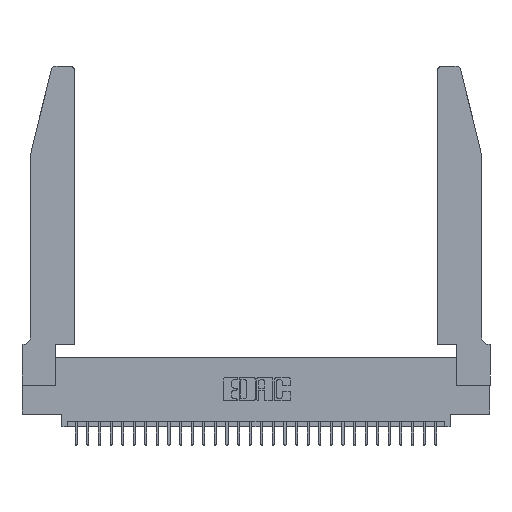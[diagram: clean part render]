
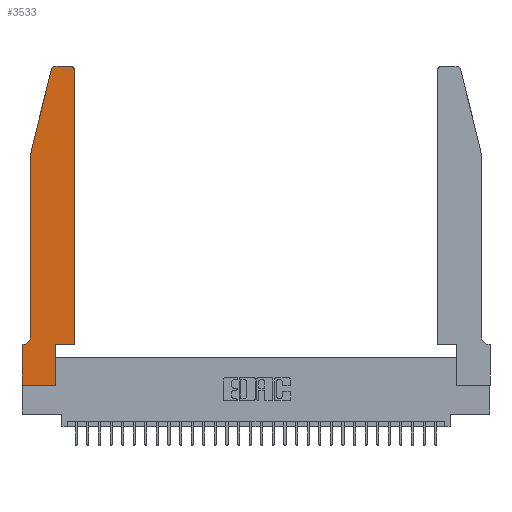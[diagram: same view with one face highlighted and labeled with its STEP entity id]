
A CAD part, top view. The second image highlights one B-rep face of the part: STEP entity #3533.
In plain terms, the highlighted planar face has unit normal (0, 0, 1).
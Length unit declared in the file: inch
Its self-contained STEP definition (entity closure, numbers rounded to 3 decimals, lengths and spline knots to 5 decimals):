
#218 = VERTEX_POINT ( 'NONE', #27734 ) ;
#499 = CARTESIAN_POINT ( 'NONE',  ( 0.4205, 2.75, 0.37 ) ) ;
#699 = ORIENTED_EDGE ( 'NONE', *, *, #30425, .T. ) ;
#1100 = CARTESIAN_POINT ( 'NONE',  ( 0., 0.35, 0.37 ) ) ;
#2359 = VECTOR ( 'NONE', #8908, 39.37008 ) ;
#2735 = CARTESIAN_POINT ( 'NONE',  ( 0.25487, 2.72718, 0.37 ) ) ;
#2744 = EDGE_CURVE ( 'NONE', #24857, #29278, #3228, .T. ) ;
#3105 = LINE ( 'NONE', #30791, #2359 ) ;
#3228 = LINE ( 'NONE', #4613, #9637 ) ;
#3513 = DIRECTION ( 'NONE',  ( 1., 0., 0. ) ) ;
#3533 = ADVANCED_FACE ( 'NONE', ( #19775 ), #13140, .T. ) ;
#3555 = EDGE_CURVE ( 'NONE', #11175, #10775, #25523, .T. ) ;
#3823 = CARTESIAN_POINT ( 'NONE',  ( 0.284, 2.72, 0.37 ) ) ;
#3853 = VECTOR ( 'NONE', #5440, 39.37008 ) ;
#3947 = VECTOR ( 'NONE', #5160, 39.37008 ) ;
#4548 = DIRECTION ( 'NONE',  ( 1., 0., 0. ) ) ;
#4613 = CARTESIAN_POINT ( 'NONE',  ( 0.2865, 0.35, 0.37 ) ) ;
#5160 = DIRECTION ( 'NONE',  ( 0., 1., 0. ) ) ;
#5346 = EDGE_CURVE ( 'NONE', #21901, #9285, #3105, .T. ) ;
#5440 = DIRECTION ( 'NONE',  ( -0.239, -0.971, 0. ) ) ;
#5837 = ORIENTED_EDGE ( 'NONE', *, *, #24663, .T. ) ;
#6046 = CARTESIAN_POINT ( 'NONE',  ( 0.0055, 0.42, 0.37 ) ) ;
#6235 = DIRECTION ( 'NONE',  ( 1., 0., 0. ) ) ;
#6561 = DIRECTION ( 'NONE',  ( -1., 0., 0. ) ) ;
#7118 = EDGE_CURVE ( 'NONE', #29278, #11805, #7823, .T. ) ;
#7313 = LINE ( 'NONE', #27795, #12979 ) ;
#7823 = LINE ( 'NONE', #28705, #19147 ) ;
#7829 = CARTESIAN_POINT ( 'NONE',  ( 0., 0., 0.37 ) ) ;
#7882 = CARTESIAN_POINT ( 'NONE',  ( 0.0755, 2., 0.37 ) ) ;
#8214 = LINE ( 'NONE', #7829, #20287 ) ;
#8465 = DIRECTION ( 'NONE',  ( -1., 0., 0. ) ) ;
#8908 = DIRECTION ( 'NONE',  ( 0., -1., 0. ) ) ;
#9285 = VERTEX_POINT ( 'NONE', #27632 ) ;
#9637 = VECTOR ( 'NONE', #21511, 39.37008 ) ;
#10223 = DIRECTION ( 'NONE',  ( 1., 0., 0. ) ) ;
#10509 = DIRECTION ( 'NONE',  ( 0., 0., 1. ) ) ;
#10563 = ORIENTED_EDGE ( 'NONE', *, *, #26636, .T. ) ;
#10751 = ORIENTED_EDGE ( 'NONE', *, *, #21285, .T. ) ;
#10775 = VERTEX_POINT ( 'NONE', #20086 ) ;
#11175 = VERTEX_POINT ( 'NONE', #16517 ) ;
#11247 = ORIENTED_EDGE ( 'NONE', *, *, #3555, .T. ) ;
#11267 = LINE ( 'NONE', #27327, #16921 ) ;
#11805 = VERTEX_POINT ( 'NONE', #21304 ) ;
#12210 = LINE ( 'NONE', #28324, #17114 ) ;
#12979 = VECTOR ( 'NONE', #13257, 39.37008 ) ;
#13085 = ORIENTED_EDGE ( 'NONE', *, *, #29826, .T. ) ;
#13140 = PLANE ( 'NONE',  #22044 ) ;
#13257 = DIRECTION ( 'NONE',  ( -1., 0., 0. ) ) ;
#13294 = CARTESIAN_POINT ( 'NONE',  ( 0.2865, 0., 0.37 ) ) ;
#14452 = EDGE_CURVE ( 'NONE', #20667, #27551, #23147, .T. ) ;
#16517 = CARTESIAN_POINT ( 'NONE',  ( 0.0755, 0.42, 0.37 ) ) ;
#16921 = VECTOR ( 'NONE', #29775, 39.37008 ) ;
#17114 = VECTOR ( 'NONE', #6561, 39.37008 ) ;
#17447 = CIRCLE ( 'NONE', #19623, 0.03 ) ;
#18001 = DIRECTION ( 'NONE',  ( 0., 0., 1. ) ) ;
#18551 = VERTEX_POINT ( 'NONE', #499 ) ;
#18901 = EDGE_CURVE ( 'NONE', #11805, #218, #29734, .T. ) ;
#19147 = VECTOR ( 'NONE', #4548, 39.37008 ) ;
#19623 = AXIS2_PLACEMENT_3D ( 'NONE', #3823, #20703, #6235 ) ;
#19775 = FACE_OUTER_BOUND ( 'NONE', #28255, .T. ) ;
#19799 = ORIENTED_EDGE ( 'NONE', *, *, #2744, .T. ) ;
#20086 = CARTESIAN_POINT ( 'NONE',  ( 0.0055, 0.35, 0.37 ) ) ;
#20287 = VECTOR ( 'NONE', #10223, 39.37008 ) ;
#20414 = AXIS2_PLACEMENT_3D ( 'NONE', #6046, #22971, #8465 ) ;
#20667 = VERTEX_POINT ( 'NONE', #2735 ) ;
#20703 = DIRECTION ( 'NONE',  ( 0., 0., 1. ) ) ;
#21044 = VERTEX_POINT ( 'NONE', #23201 ) ;
#21285 = EDGE_CURVE ( 'NONE', #18551, #21044, #12210, .T. ) ;
#21304 = CARTESIAN_POINT ( 'NONE',  ( 0.4505, 0.35, 0.37 ) ) ;
#21511 = DIRECTION ( 'NONE',  ( 0., 1., 0. ) ) ;
#21901 = VERTEX_POINT ( 'NONE', #25727 ) ;
#22044 = AXIS2_PLACEMENT_3D ( 'NONE', #1100, #18001, #3513 ) ;
#22444 = AXIS2_PLACEMENT_3D ( 'NONE', #25043, #10509, #27498 ) ;
#22971 = DIRECTION ( 'NONE',  ( 0., 0., -1. ) ) ;
#23147 = LINE ( 'NONE', #7882, #3853 ) ;
#23201 = CARTESIAN_POINT ( 'NONE',  ( 0.284, 2.75, 0.37 ) ) ;
#24405 = CARTESIAN_POINT ( 'NONE',  ( 0.4505, 0.35, 0.37 ) ) ;
#24663 = EDGE_CURVE ( 'NONE', #9285, #24857, #8214, .T. ) ;
#24857 = VERTEX_POINT ( 'NONE', #13294 ) ;
#25043 = CARTESIAN_POINT ( 'NONE',  ( 0.4205, 2.72, 0.37 ) ) ;
#25523 = CIRCLE ( 'NONE', #20414, 0.07 ) ;
#25707 = CARTESIAN_POINT ( 'NONE',  ( 0.2865, 0.35, 0.37 ) ) ;
#25727 = CARTESIAN_POINT ( 'NONE',  ( 0., 0.35, 0.37 ) ) ;
#26636 = EDGE_CURVE ( 'NONE', #27551, #11175, #11267, .T. ) ;
#26815 = ORIENTED_EDGE ( 'NONE', *, *, #31174, .T. ) ;
#27327 = CARTESIAN_POINT ( 'NONE',  ( 0.0755, 2., 0.37 ) ) ;
#27498 = DIRECTION ( 'NONE',  ( 1., 0., 0. ) ) ;
#27551 = VERTEX_POINT ( 'NONE', #28472 ) ;
#27632 = CARTESIAN_POINT ( 'NONE',  ( 0., 0., 0.37 ) ) ;
#27734 = CARTESIAN_POINT ( 'NONE',  ( 0.4505, 2.72, 0.37 ) ) ;
#27795 = CARTESIAN_POINT ( 'NONE',  ( 0.0755, 0.35, 0.37 ) ) ;
#27957 = ORIENTED_EDGE ( 'NONE', *, *, #18901, .T. ) ;
#28255 = EDGE_LOOP ( 'NONE', ( #10751, #26815, #28413, #10563, #11247, #13085, #31333, #5837, #19799, #29565, #27957, #699 ) ) ;
#28324 = CARTESIAN_POINT ( 'NONE',  ( 0.2605, 2.75, 0.37 ) ) ;
#28413 = ORIENTED_EDGE ( 'NONE', *, *, #14452, .T. ) ;
#28472 = CARTESIAN_POINT ( 'NONE',  ( 0.0755, 2., 0.37 ) ) ;
#28531 = CIRCLE ( 'NONE', #22444, 0.03 ) ;
#28705 = CARTESIAN_POINT ( 'NONE',  ( 0.4505, 0.35, 0.37 ) ) ;
#29278 = VERTEX_POINT ( 'NONE', #25707 ) ;
#29565 = ORIENTED_EDGE ( 'NONE', *, *, #7118, .T. ) ;
#29734 = LINE ( 'NONE', #24405, #3947 ) ;
#29775 = DIRECTION ( 'NONE',  ( 0., -1., 0. ) ) ;
#29826 = EDGE_CURVE ( 'NONE', #10775, #21901, #7313, .T. ) ;
#30425 = EDGE_CURVE ( 'NONE', #218, #18551, #28531, .T. ) ;
#30791 = CARTESIAN_POINT ( 'NONE',  ( 0., 0., 0.37 ) ) ;
#31174 = EDGE_CURVE ( 'NONE', #21044, #20667, #17447, .T. ) ;
#31333 = ORIENTED_EDGE ( 'NONE', *, *, #5346, .T. ) ;
